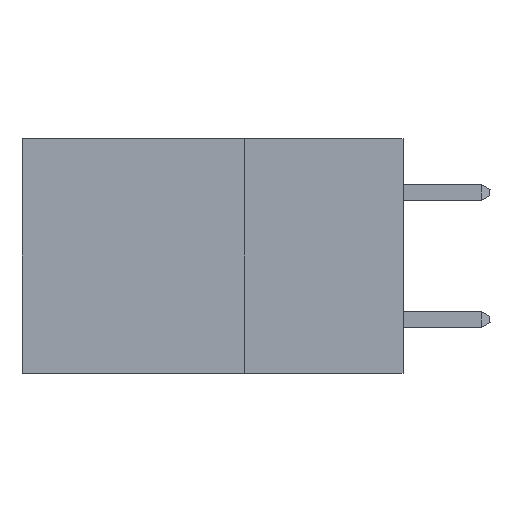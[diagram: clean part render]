
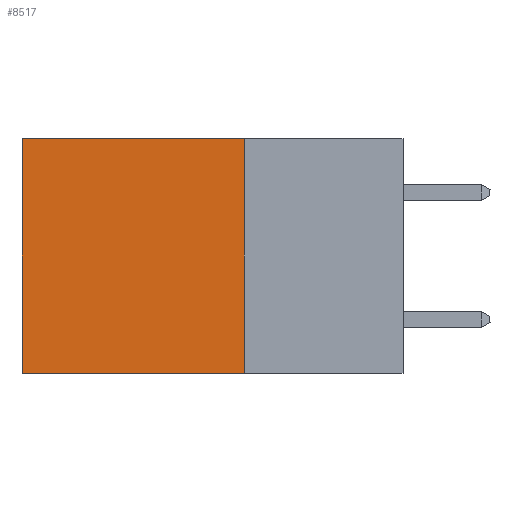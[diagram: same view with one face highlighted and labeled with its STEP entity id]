
A CAD part, left-side view. The second image highlights one B-rep face of the part: STEP entity #8517.
In plain terms, the highlighted planar face has unit normal (-1, 0, 0).
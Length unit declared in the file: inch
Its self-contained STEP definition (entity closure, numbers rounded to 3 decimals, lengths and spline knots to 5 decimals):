
#273 = CARTESIAN_POINT ( 'NONE',  ( 0.2875, 0.25, 0. ) ) ;
#372 = DIRECTION ( 'NONE',  ( 1., 0., 0. ) ) ;
#1029 = CARTESIAN_POINT ( 'NONE',  ( 0.2875, 0.6, 0. ) ) ;
#1300 = ORIENTED_EDGE ( 'NONE', *, *, #10524, .F. ) ;
#1448 = VERTEX_POINT ( 'NONE', #4187 ) ;
#1575 = DIRECTION ( 'NONE',  ( 0., 1., 0. ) ) ;
#1596 = EDGE_CURVE ( 'NONE', #8830, #11127, #11920, .T. ) ;
#1995 = FACE_OUTER_BOUND ( 'NONE', #7977, .T. ) ;
#2186 = CARTESIAN_POINT ( 'NONE',  ( 0.2875, 0.6, 0. ) ) ;
#2654 = VECTOR ( 'NONE', #1575, 39.37008 ) ;
#3013 = DIRECTION ( 'NONE',  ( 0., 0., -1. ) ) ;
#4187 = CARTESIAN_POINT ( 'NONE',  ( 0.2875, 0.25, -0.37 ) ) ;
#4434 = ORIENTED_EDGE ( 'NONE', *, *, #1596, .T. ) ;
#5149 = DIRECTION ( 'NONE',  ( 0., 1., 0. ) ) ;
#5160 = CARTESIAN_POINT ( 'NONE',  ( 0.2875, 0.25, 0. ) ) ;
#5232 = VERTEX_POINT ( 'NONE', #10783 ) ;
#5676 = VECTOR ( 'NONE', #5149, 39.37008 ) ;
#6278 = CARTESIAN_POINT ( 'NONE',  ( 0.2875, 0.25, 0. ) ) ;
#7608 = CARTESIAN_POINT ( 'NONE',  ( 0.2875, 0.25, -0.37 ) ) ;
#7703 = EDGE_CURVE ( 'NONE', #5232, #1448, #11428, .T. ) ;
#7977 = EDGE_LOOP ( 'NONE', ( #4434, #1300, #11297, #9572 ) ) ;
#8517 = ADVANCED_FACE ( 'NONE', ( #1995 ), #13852, .F. ) ;
#8552 = VECTOR ( 'NONE', #9052, 39.37008 ) ;
#8830 = VERTEX_POINT ( 'NONE', #2186 ) ;
#9052 = DIRECTION ( 'NONE',  ( 0., 0., -1. ) ) ;
#9572 = ORIENTED_EDGE ( 'NONE', *, *, #11921, .T. ) ;
#9701 = LINE ( 'NONE', #6278, #5676 ) ;
#10524 = EDGE_CURVE ( 'NONE', #1448, #11127, #11716, .T. ) ;
#10783 = CARTESIAN_POINT ( 'NONE',  ( 0.2875, 0.25, 0. ) ) ;
#11127 = VERTEX_POINT ( 'NONE', #13373 ) ;
#11297 = ORIENTED_EDGE ( 'NONE', *, *, #7703, .F. ) ;
#11428 = LINE ( 'NONE', #5160, #14089 ) ;
#11662 = DIRECTION ( 'NONE',  ( 0., 0., -1. ) ) ;
#11716 = LINE ( 'NONE', #7608, #2654 ) ;
#11920 = LINE ( 'NONE', #1029, #8552 ) ;
#11921 = EDGE_CURVE ( 'NONE', #5232, #8830, #9701, .T. ) ;
#12616 = AXIS2_PLACEMENT_3D ( 'NONE', #273, #372, #11662 ) ;
#13373 = CARTESIAN_POINT ( 'NONE',  ( 0.2875, 0.6, -0.37 ) ) ;
#13852 = PLANE ( 'NONE',  #12616 ) ;
#14089 = VECTOR ( 'NONE', #3013, 39.37008 ) ;
